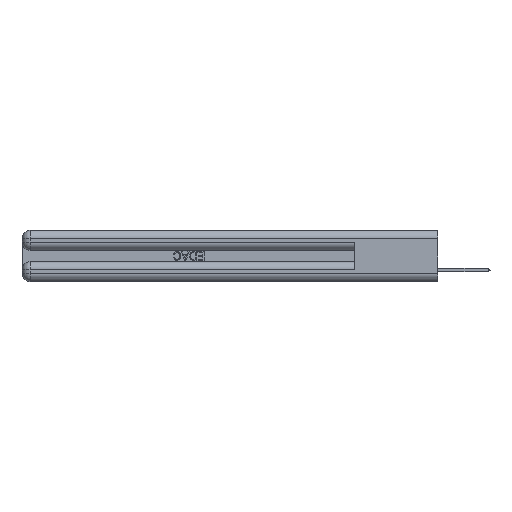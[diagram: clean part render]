
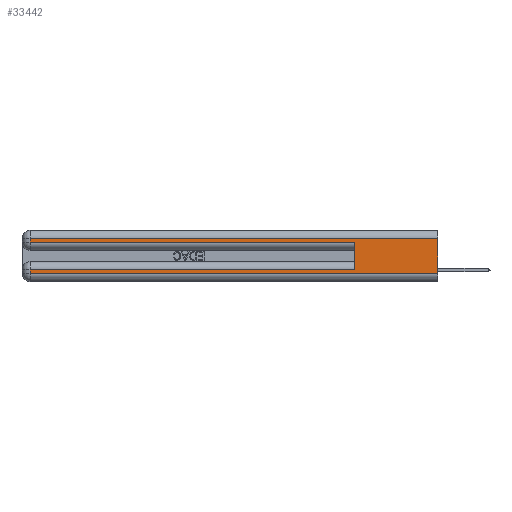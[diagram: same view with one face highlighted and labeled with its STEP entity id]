
A CAD part, left-side view. The second image highlights one B-rep face of the part: STEP entity #33442.
In plain terms, the highlighted planar face has unit normal (-1, 0, 0).
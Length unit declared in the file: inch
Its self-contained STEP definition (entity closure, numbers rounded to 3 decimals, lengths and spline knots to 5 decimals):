
#172 = CARTESIAN_POINT ( 'NONE',  ( 0., 2.94, 0.285 ) ) ;
#232 = VECTOR ( 'NONE', #24180, 39.37008 ) ;
#580 = ORIENTED_EDGE ( 'NONE', *, *, #1843, .T. ) ;
#774 = EDGE_LOOP ( 'NONE', ( #37310, #8380, #40374, #40140, #22018, #37451, #22194, #580 ) ) ;
#927 = DIRECTION ( 'NONE',  ( 1., 0., 0. ) ) ;
#1513 = LINE ( 'NONE', #30171, #39135 ) ;
#1843 = EDGE_CURVE ( 'NONE', #35382, #7880, #38822, .T. ) ;
#3611 = CARTESIAN_POINT ( 'NONE',  ( 0., 0., 0.31 ) ) ;
#5349 = EDGE_CURVE ( 'NONE', #17603, #6792, #24956, .T. ) ;
#5945 = CARTESIAN_POINT ( 'NONE',  ( 0., 0.6, 0.085 ) ) ;
#6479 = VERTEX_POINT ( 'NONE', #172 ) ;
#6503 = DIRECTION ( 'NONE',  ( 0., 1., 0. ) ) ;
#6792 = VERTEX_POINT ( 'NONE', #30570 ) ;
#7880 = VERTEX_POINT ( 'NONE', #8962 ) ;
#8187 = CARTESIAN_POINT ( 'NONE',  ( 0., 0., 0.37 ) ) ;
#8380 = ORIENTED_EDGE ( 'NONE', *, *, #5349, .T. ) ;
#8431 = DIRECTION ( 'NONE',  ( 0., 0., -1. ) ) ;
#8962 = CARTESIAN_POINT ( 'NONE',  ( 0., 0., 0.06 ) ) ;
#10077 = DIRECTION ( 'NONE',  ( 0., 0., -1. ) ) ;
#11983 = AXIS2_PLACEMENT_3D ( 'NONE', #31816, #927, #28710 ) ;
#12293 = CARTESIAN_POINT ( 'NONE',  ( 0., 2.94, 0.37 ) ) ;
#13053 = CARTESIAN_POINT ( 'NONE',  ( 0., 0., 0.31 ) ) ;
#13219 = VERTEX_POINT ( 'NONE', #16402 ) ;
#14064 = DIRECTION ( 'NONE',  ( 0., 0., 1. ) ) ;
#14945 = LINE ( 'NONE', #21020, #232 ) ;
#15127 = VECTOR ( 'NONE', #6503, 39.37008 ) ;
#16402 = CARTESIAN_POINT ( 'NONE',  ( 0., 2.94, 0.085 ) ) ;
#17164 = CARTESIAN_POINT ( 'NONE',  ( 0., 0., 0.06 ) ) ;
#17603 = VERTEX_POINT ( 'NONE', #3611 ) ;
#18468 = EDGE_CURVE ( 'NONE', #6479, #19329, #14945, .T. ) ;
#19329 = VERTEX_POINT ( 'NONE', #34096 ) ;
#20716 = VECTOR ( 'NONE', #10077, 39.37008 ) ;
#21020 = CARTESIAN_POINT ( 'NONE',  ( 0., 0., 0.285 ) ) ;
#21779 = VECTOR ( 'NONE', #24343, 39.37008 ) ;
#22018 = ORIENTED_EDGE ( 'NONE', *, *, #27764, .F. ) ;
#22194 = ORIENTED_EDGE ( 'NONE', *, *, #36309, .T. ) ;
#22554 = PLANE ( 'NONE',  #11983 ) ;
#23203 = EDGE_CURVE ( 'NONE', #17603, #7880, #34445, .T. ) ;
#24180 = DIRECTION ( 'NONE',  ( 0., -1., 0. ) ) ;
#24343 = DIRECTION ( 'NONE',  ( 0., 0., -1. ) ) ;
#24956 = LINE ( 'NONE', #13053, #15127 ) ;
#25165 = EDGE_CURVE ( 'NONE', #6792, #6479, #1513, .T. ) ;
#27531 = CARTESIAN_POINT ( 'NONE',  ( 0., 0., 0.085 ) ) ;
#27764 = EDGE_CURVE ( 'NONE', #34438, #19329, #33467, .T. ) ;
#28710 = DIRECTION ( 'NONE',  ( 0., 0., -1. ) ) ;
#30012 = LINE ( 'NONE', #12293, #20716 ) ;
#30171 = CARTESIAN_POINT ( 'NONE',  ( 0., 2.94, 0.37 ) ) ;
#30570 = CARTESIAN_POINT ( 'NONE',  ( 0., 2.94, 0.31 ) ) ;
#31039 = VECTOR ( 'NONE', #38996, 39.37008 ) ;
#31816 = CARTESIAN_POINT ( 'NONE',  ( 0., 0., 0.37 ) ) ;
#32631 = VECTOR ( 'NONE', #33622, 39.37008 ) ;
#33096 = FACE_OUTER_BOUND ( 'NONE', #774, .T. ) ;
#33202 = EDGE_CURVE ( 'NONE', #34438, #13219, #37047, .T. ) ;
#33442 = ADVANCED_FACE ( 'NONE', ( #33096 ), #22554, .F. ) ;
#33467 = LINE ( 'NONE', #35776, #37401 ) ;
#33622 = DIRECTION ( 'NONE',  ( 0., 1., 0. ) ) ;
#34096 = CARTESIAN_POINT ( 'NONE',  ( 0., 0.6, 0.285 ) ) ;
#34438 = VERTEX_POINT ( 'NONE', #5945 ) ;
#34445 = LINE ( 'NONE', #8187, #21779 ) ;
#35382 = VERTEX_POINT ( 'NONE', #36937 ) ;
#35776 = CARTESIAN_POINT ( 'NONE',  ( 0., 0.6, 0.145 ) ) ;
#36309 = EDGE_CURVE ( 'NONE', #13219, #35382, #30012, .T. ) ;
#36937 = CARTESIAN_POINT ( 'NONE',  ( 0., 2.94, 0.06 ) ) ;
#37047 = LINE ( 'NONE', #27531, #32631 ) ;
#37310 = ORIENTED_EDGE ( 'NONE', *, *, #23203, .F. ) ;
#37401 = VECTOR ( 'NONE', #14064, 39.37008 ) ;
#37451 = ORIENTED_EDGE ( 'NONE', *, *, #33202, .T. ) ;
#38822 = LINE ( 'NONE', #17164, #31039 ) ;
#38996 = DIRECTION ( 'NONE',  ( 0., -1., 0. ) ) ;
#39135 = VECTOR ( 'NONE', #8431, 39.37008 ) ;
#40140 = ORIENTED_EDGE ( 'NONE', *, *, #18468, .T. ) ;
#40374 = ORIENTED_EDGE ( 'NONE', *, *, #25165, .T. ) ;
